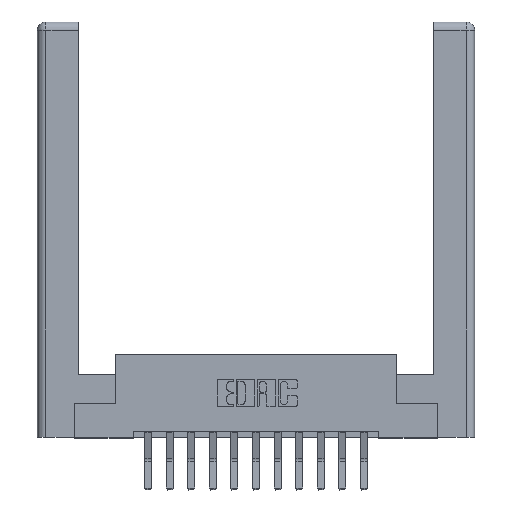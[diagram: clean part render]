
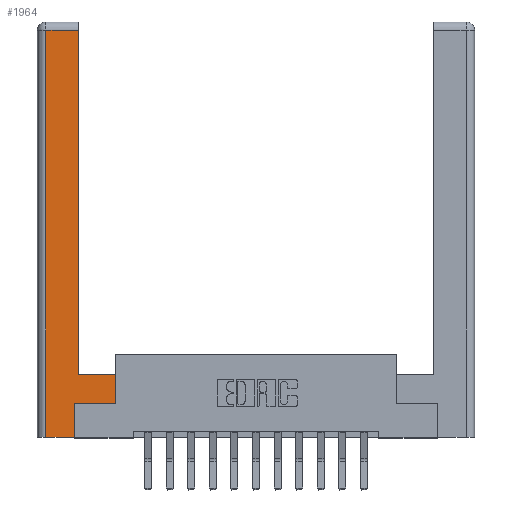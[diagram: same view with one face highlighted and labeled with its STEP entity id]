
A CAD part, top view. The second image highlights one B-rep face of the part: STEP entity #1964.
In plain terms, the highlighted planar face has unit normal (0, 0, 1).
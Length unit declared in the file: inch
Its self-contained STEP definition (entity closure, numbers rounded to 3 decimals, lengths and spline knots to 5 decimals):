
#387 = DIRECTION ( 'NONE',  ( 1., 0., 0. ) ) ;
#499 = CARTESIAN_POINT ( 'NONE',  ( 0.0615, 2.94, 0. ) ) ;
#526 = CARTESIAN_POINT ( 'NONE',  ( 0.295, 0.45, 0. ) ) ;
#596 = ORIENTED_EDGE ( 'NONE', *, *, #3159, .T. ) ;
#1275 = EDGE_CURVE ( 'NONE', #3022, #11438, #1432, .T. ) ;
#1277 = VERTEX_POINT ( 'NONE', #526 ) ;
#1432 = LINE ( 'NONE', #2892, #5306 ) ;
#1764 = VECTOR ( 'NONE', #14472, 39.37008 ) ;
#1782 = VERTEX_POINT ( 'NONE', #2665 ) ;
#1964 = ADVANCED_FACE ( 'NONE', ( #5309 ), #12696, .F. ) ;
#2069 = ORIENTED_EDGE ( 'NONE', *, *, #8350, .T. ) ;
#2205 = DIRECTION ( 'NONE',  ( 1., 0., 0. ) ) ;
#2528 = CARTESIAN_POINT ( 'NONE',  ( 0.265, 0., 0. ) ) ;
#2665 = CARTESIAN_POINT ( 'NONE',  ( 0.565, 0.245, 0. ) ) ;
#2755 = EDGE_CURVE ( 'NONE', #1277, #3022, #6018, .T. ) ;
#2892 = CARTESIAN_POINT ( 'NONE',  ( 0.0615, 2.94, 0. ) ) ;
#3022 = VERTEX_POINT ( 'NONE', #9491 ) ;
#3159 = EDGE_CURVE ( 'NONE', #14642, #8711, #5833, .T. ) ;
#3281 = LINE ( 'NONE', #4590, #10062 ) ;
#3462 = VECTOR ( 'NONE', #10209, 39.37008 ) ;
#3473 = LINE ( 'NONE', #12632, #4361 ) ;
#3552 = DIRECTION ( 'NONE',  ( 0., 1., 0. ) ) ;
#3775 = CARTESIAN_POINT ( 'NONE',  ( 0.0615, 0., 0. ) ) ;
#4095 = CARTESIAN_POINT ( 'NONE',  ( 0.295, 0.45, 0. ) ) ;
#4107 = AXIS2_PLACEMENT_3D ( 'NONE', #9222, #5742, #6758 ) ;
#4361 = VECTOR ( 'NONE', #7872, 39.37008 ) ;
#4590 = CARTESIAN_POINT ( 'NONE',  ( 0.565, 0.245, 0. ) ) ;
#5091 = CARTESIAN_POINT ( 'NONE',  ( 0.265, 0., 0. ) ) ;
#5221 = VERTEX_POINT ( 'NONE', #8680 ) ;
#5293 = LINE ( 'NONE', #3775, #1764 ) ;
#5306 = VECTOR ( 'NONE', #14760, 39.37008 ) ;
#5309 = FACE_OUTER_BOUND ( 'NONE', #11051, .T. ) ;
#5742 = DIRECTION ( 'NONE',  ( 0., 0., -1. ) ) ;
#5833 = LINE ( 'NONE', #5091, #11318 ) ;
#6018 = LINE ( 'NONE', #12754, #3462 ) ;
#6225 = LINE ( 'NONE', #14206, #9143 ) ;
#6758 = DIRECTION ( 'NONE',  ( -1., 0., 0. ) ) ;
#6990 = ORIENTED_EDGE ( 'NONE', *, *, #13855, .T. ) ;
#7872 = DIRECTION ( 'NONE',  ( 0., 1., 0. ) ) ;
#8350 = EDGE_CURVE ( 'NONE', #5221, #1277, #11362, .T. ) ;
#8680 = CARTESIAN_POINT ( 'NONE',  ( 0.565, 0.45, 0. ) ) ;
#8711 = VERTEX_POINT ( 'NONE', #2528 ) ;
#8751 = ORIENTED_EDGE ( 'NONE', *, *, #1275, .T. ) ;
#8778 = EDGE_CURVE ( 'NONE', #1782, #5221, #6225, .T. ) ;
#9143 = VECTOR ( 'NONE', #3552, 39.37008 ) ;
#9222 = CARTESIAN_POINT ( 'NONE',  ( 0., 0., 0. ) ) ;
#9286 = ORIENTED_EDGE ( 'NONE', *, *, #8778, .T. ) ;
#9479 = EDGE_CURVE ( 'NONE', #11438, #14642, #5293, .T. ) ;
#9491 = CARTESIAN_POINT ( 'NONE',  ( 0.295, 2.94, 0. ) ) ;
#9493 = ORIENTED_EDGE ( 'NONE', *, *, #2755, .T. ) ;
#9838 = DIRECTION ( 'NONE',  ( -1., 0., 0. ) ) ;
#10062 = VECTOR ( 'NONE', #2205, 39.37008 ) ;
#10209 = DIRECTION ( 'NONE',  ( 0., 1., 0. ) ) ;
#11051 = EDGE_LOOP ( 'NONE', ( #9493, #8751, #13947, #596, #6990, #13089, #9286, #2069 ) ) ;
#11318 = VECTOR ( 'NONE', #387, 39.37008 ) ;
#11362 = LINE ( 'NONE', #4095, #15092 ) ;
#11438 = VERTEX_POINT ( 'NONE', #499 ) ;
#11712 = VERTEX_POINT ( 'NONE', #12274 ) ;
#12190 = CARTESIAN_POINT ( 'NONE',  ( 0.0615, 0., 0. ) ) ;
#12274 = CARTESIAN_POINT ( 'NONE',  ( 0.265, 0.245, 0. ) ) ;
#12632 = CARTESIAN_POINT ( 'NONE',  ( 0.265, 0.245, 0. ) ) ;
#12696 = PLANE ( 'NONE',  #4107 ) ;
#12754 = CARTESIAN_POINT ( 'NONE',  ( 0.295, 3., 0. ) ) ;
#13089 = ORIENTED_EDGE ( 'NONE', *, *, #13214, .T. ) ;
#13214 = EDGE_CURVE ( 'NONE', #11712, #1782, #3281, .T. ) ;
#13855 = EDGE_CURVE ( 'NONE', #8711, #11712, #3473, .T. ) ;
#13947 = ORIENTED_EDGE ( 'NONE', *, *, #9479, .T. ) ;
#14206 = CARTESIAN_POINT ( 'NONE',  ( 0.565, 0.45, 0. ) ) ;
#14472 = DIRECTION ( 'NONE',  ( 0., -1., 0. ) ) ;
#14642 = VERTEX_POINT ( 'NONE', #12190 ) ;
#14760 = DIRECTION ( 'NONE',  ( -1., 0., 0. ) ) ;
#15092 = VECTOR ( 'NONE', #9838, 39.37008 ) ;
